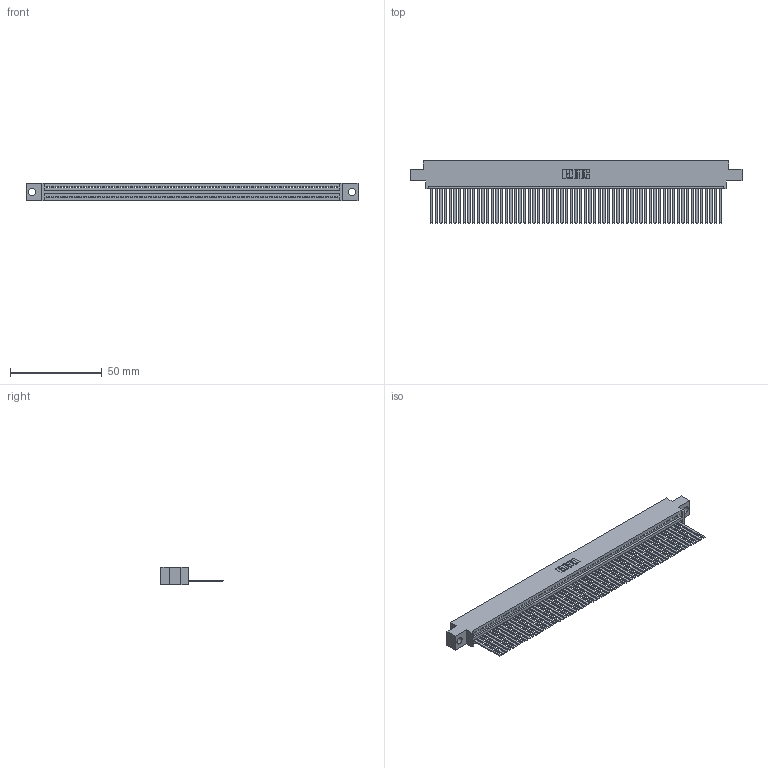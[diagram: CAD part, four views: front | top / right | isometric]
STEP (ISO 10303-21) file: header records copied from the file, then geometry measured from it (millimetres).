
FILE_DESCRIPTION (( 'STEP AP203' ), '1' );
FILE_NAME ('395-063-544-604.STEP', '2019-10-24T23:26:21', ( '' ), ( '' ), 'SwSTEP 2.0', 'SolidWorks 2016', '' );
FILE_SCHEMA (( 'CONFIG_CONTROL_DESIGN' ));
Length unit declared in the file: inch
Products named in the file (3): 395-063-544-604; 345-292-001_345-293-144; 345 Part_0.170 Offset - 0.156 Dia-TH
Assembly tree (64 placements, depth 2):
  395-063-544-604
    345 Part_0.170 Offset - 0.156 Dia-TH
    345-292-001_345-293-144  x63
Bounding box: 181.23 x 33.96 x 9.4 mm (x, y, z)
Volume: 17913.7 mm3; surface area: 26216.8 mm2
Topology: 64 solids, 64 shells, 3406 faces, 10307 edges, 6786 vertices
Faces by surface type: plane 2352, cylinder 1054
Entity records: 44539 total; most frequent: CARTESIAN_POINT 7721, ORIENTED_EDGE 7718, DIRECTION 6709, EDGE_CURVE 3859, LINE 3479, VECTOR 3479, VERTEX_POINT 2570, AXIS2_PLACEMENT_3D 1615
